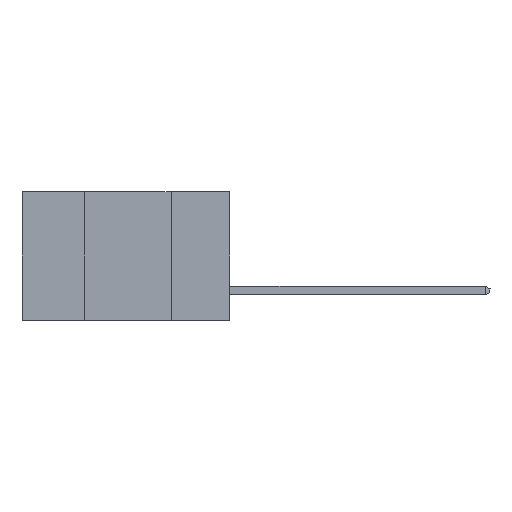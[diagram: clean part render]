
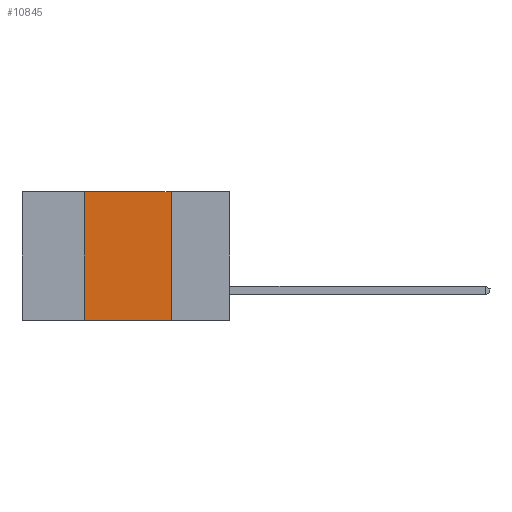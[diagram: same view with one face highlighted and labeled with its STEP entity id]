
A CAD part, left-side view. The second image highlights one B-rep face of the part: STEP entity #10845.
In plain terms, the highlighted planar face has unit normal (-1, 0, 0).
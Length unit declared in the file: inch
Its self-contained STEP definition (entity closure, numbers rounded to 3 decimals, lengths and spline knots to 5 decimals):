
#50 = VERTEX_POINT ( 'NONE', #10654 ) ;
#221 = VECTOR ( 'NONE', #9753, 39.37008 ) ;
#492 = CARTESIAN_POINT ( 'NONE',  ( 0., 0.6, -0.37 ) ) ;
#807 = PLANE ( 'NONE',  #7413 ) ;
#948 = CARTESIAN_POINT ( 'NONE',  ( 0., 0.42, 0. ) ) ;
#1741 = DIRECTION ( 'NONE',  ( 1., 0., 0. ) ) ;
#1825 = LINE ( 'NONE', #9203, #4390 ) ;
#1963 = VERTEX_POINT ( 'NONE', #3720 ) ;
#2209 = CARTESIAN_POINT ( 'NONE',  ( 0., 0.42, -0.37 ) ) ;
#2374 = DIRECTION ( 'NONE',  ( 0., -1., 0. ) ) ;
#3720 = CARTESIAN_POINT ( 'NONE',  ( 0., 0.42, -0.37 ) ) ;
#3762 = EDGE_CURVE ( 'NONE', #50, #4502, #11410, .T. ) ;
#3977 = ORIENTED_EDGE ( 'NONE', *, *, #10286, .F. ) ;
#4390 = VECTOR ( 'NONE', #5719, 39.37008 ) ;
#4502 = VERTEX_POINT ( 'NONE', #7771 ) ;
#5204 = VERTEX_POINT ( 'NONE', #948 ) ;
#5719 = DIRECTION ( 'NONE',  ( 0., -1., 0. ) ) ;
#5889 = VECTOR ( 'NONE', #7489, 39.37008 ) ;
#5898 = VECTOR ( 'NONE', #2374, 39.37008 ) ;
#5988 = LINE ( 'NONE', #492, #5898 ) ;
#6927 = ORIENTED_EDGE ( 'NONE', *, *, #3762, .F. ) ;
#7413 = AXIS2_PLACEMENT_3D ( 'NONE', #11599, #1741, #8015 ) ;
#7489 = DIRECTION ( 'NONE',  ( 0., 0., 1. ) ) ;
#7771 = CARTESIAN_POINT ( 'NONE',  ( 0., 0.17, -0.37 ) ) ;
#8015 = DIRECTION ( 'NONE',  ( 0., 0., -1. ) ) ;
#8815 = CARTESIAN_POINT ( 'NONE',  ( 0., 0.17, -0.37 ) ) ;
#8888 = FACE_OUTER_BOUND ( 'NONE', #9789, .T. ) ;
#9056 = EDGE_CURVE ( 'NONE', #1963, #4502, #5988, .T. ) ;
#9203 = CARTESIAN_POINT ( 'NONE',  ( 0., 0.6, 0. ) ) ;
#9378 = LINE ( 'NONE', #2209, #5889 ) ;
#9490 = ORIENTED_EDGE ( 'NONE', *, *, #10603, .F. ) ;
#9753 = DIRECTION ( 'NONE',  ( 0., 0., -1. ) ) ;
#9789 = EDGE_LOOP ( 'NONE', ( #6927, #9490, #3977, #9802 ) ) ;
#9802 = ORIENTED_EDGE ( 'NONE', *, *, #9056, .T. ) ;
#10286 = EDGE_CURVE ( 'NONE', #1963, #5204, #9378, .T. ) ;
#10603 = EDGE_CURVE ( 'NONE', #5204, #50, #1825, .T. ) ;
#10654 = CARTESIAN_POINT ( 'NONE',  ( 0., 0.17, 0. ) ) ;
#10845 = ADVANCED_FACE ( 'NONE', ( #8888 ), #807, .F. ) ;
#11410 = LINE ( 'NONE', #8815, #221 ) ;
#11599 = CARTESIAN_POINT ( 'NONE',  ( 0., 0.6, 0. ) ) ;
